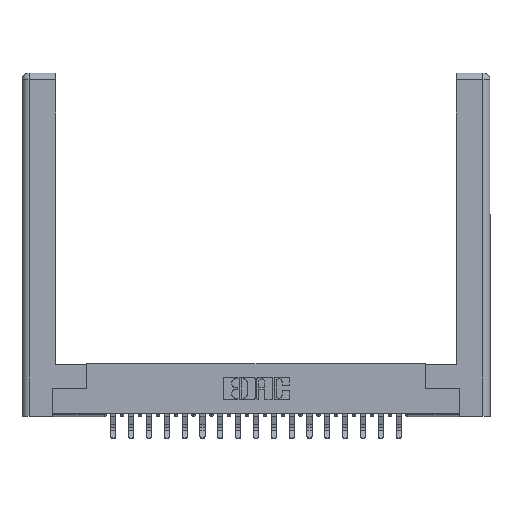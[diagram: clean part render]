
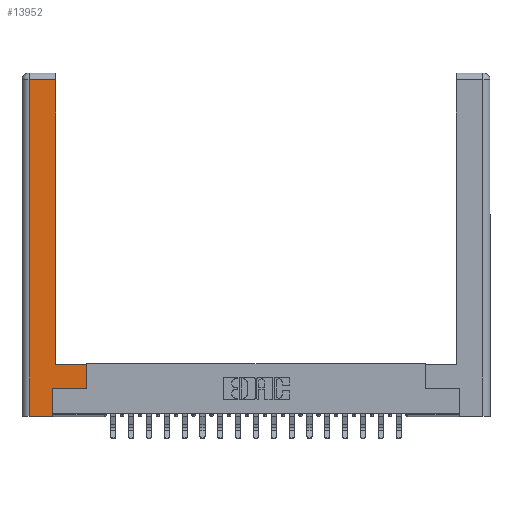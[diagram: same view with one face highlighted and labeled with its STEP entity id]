
A CAD part, top view. The second image highlights one B-rep face of the part: STEP entity #13952.
In plain terms, the highlighted planar face has unit normal (0, 0, 1).
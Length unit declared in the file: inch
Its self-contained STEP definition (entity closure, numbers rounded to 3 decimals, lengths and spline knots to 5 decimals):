
#21 = EDGE_CURVE ( 'NONE', #19868, #20368, #8283, .T. ) ;
#364 = DIRECTION ( 'NONE',  ( -1., 0., 0. ) ) ;
#647 = CARTESIAN_POINT ( 'NONE',  ( 0.0615, 0., 0. ) ) ;
#797 = ORIENTED_EDGE ( 'NONE', *, *, #3730, .T. ) ;
#887 = DIRECTION ( 'NONE',  ( 0., -1., 0. ) ) ;
#927 = ORIENTED_EDGE ( 'NONE', *, *, #7291, .T. ) ;
#1254 = EDGE_CURVE ( 'NONE', #12085, #10074, #23178, .T. ) ;
#1780 = CARTESIAN_POINT ( 'NONE',  ( 0.565, 0.45, 0. ) ) ;
#2742 = ORIENTED_EDGE ( 'NONE', *, *, #9369, .T. ) ;
#2904 = CARTESIAN_POINT ( 'NONE',  ( 0.295, 3., 0. ) ) ;
#3161 = DIRECTION ( 'NONE',  ( 0., 1., 0. ) ) ;
#3313 = CARTESIAN_POINT ( 'NONE',  ( 0.295, 2.94, 0. ) ) ;
#3516 = CARTESIAN_POINT ( 'NONE',  ( 0.0615, 0., 0. ) ) ;
#3673 = LINE ( 'NONE', #7377, #7491 ) ;
#3729 = EDGE_CURVE ( 'NONE', #15984, #19868, #7924, .T. ) ;
#3730 = EDGE_CURVE ( 'NONE', #20303, #15984, #16678, .T. ) ;
#4463 = CARTESIAN_POINT ( 'NONE',  ( 0.265, 0.245, 0. ) ) ;
#4568 = VECTOR ( 'NONE', #23417, 39.37008 ) ;
#6004 = CARTESIAN_POINT ( 'NONE',  ( 0., 0., 0. ) ) ;
#6330 = CARTESIAN_POINT ( 'NONE',  ( 0.265, 0., 0. ) ) ;
#7291 = EDGE_CURVE ( 'NONE', #19706, #12085, #3673, .T. ) ;
#7377 = CARTESIAN_POINT ( 'NONE',  ( 0.265, 0.245, 0. ) ) ;
#7491 = VECTOR ( 'NONE', #22975, 39.37008 ) ;
#7568 = CARTESIAN_POINT ( 'NONE',  ( 0.565, 0.245, 0. ) ) ;
#7638 = DIRECTION ( 'NONE',  ( 1., 0., 0. ) ) ;
#7924 = LINE ( 'NONE', #10699, #23725 ) ;
#8283 = LINE ( 'NONE', #647, #16761 ) ;
#9369 = EDGE_CURVE ( 'NONE', #19134, #20303, #10559, .T. ) ;
#9466 = VECTOR ( 'NONE', #23422, 39.37008 ) ;
#9944 = VECTOR ( 'NONE', #3161, 39.37008 ) ;
#9997 = EDGE_CURVE ( 'NONE', #20368, #19706, #22728, .T. ) ;
#10031 = LINE ( 'NONE', #23668, #9466 ) ;
#10074 = VERTEX_POINT ( 'NONE', #16698 ) ;
#10559 = LINE ( 'NONE', #20299, #12303 ) ;
#10699 = CARTESIAN_POINT ( 'NONE',  ( 0.0615, 2.94, 0. ) ) ;
#10972 = DIRECTION ( 'NONE',  ( -1., 0., 0. ) ) ;
#11454 = DIRECTION ( 'NONE',  ( 0., 0., -1. ) ) ;
#11776 = PLANE ( 'NONE',  #24151 ) ;
#12085 = VERTEX_POINT ( 'NONE', #4463 ) ;
#12303 = VECTOR ( 'NONE', #10972, 39.37008 ) ;
#12710 = CARTESIAN_POINT ( 'NONE',  ( 0.0615, 2.94, 0. ) ) ;
#13183 = VECTOR ( 'NONE', #7638, 39.37008 ) ;
#13471 = ORIENTED_EDGE ( 'NONE', *, *, #1254, .T. ) ;
#13952 = ADVANCED_FACE ( 'NONE', ( #21368 ), #11776, .F. ) ;
#15962 = ORIENTED_EDGE ( 'NONE', *, *, #18430, .T. ) ;
#15984 = VERTEX_POINT ( 'NONE', #3313 ) ;
#16678 = LINE ( 'NONE', #2904, #9944 ) ;
#16698 = CARTESIAN_POINT ( 'NONE',  ( 0.565, 0.245, 0. ) ) ;
#16761 = VECTOR ( 'NONE', #887, 39.37008 ) ;
#17154 = CARTESIAN_POINT ( 'NONE',  ( 0.265, 0., 0. ) ) ;
#18430 = EDGE_CURVE ( 'NONE', #10074, #19134, #10031, .T. ) ;
#19134 = VERTEX_POINT ( 'NONE', #1780 ) ;
#19706 = VERTEX_POINT ( 'NONE', #17154 ) ;
#19868 = VERTEX_POINT ( 'NONE', #12710 ) ;
#20299 = CARTESIAN_POINT ( 'NONE',  ( 0.295, 0.45, 0. ) ) ;
#20303 = VERTEX_POINT ( 'NONE', #21862 ) ;
#20368 = VERTEX_POINT ( 'NONE', #3516 ) ;
#21368 = FACE_OUTER_BOUND ( 'NONE', #24258, .T. ) ;
#21815 = ORIENTED_EDGE ( 'NONE', *, *, #9997, .T. ) ;
#21862 = CARTESIAN_POINT ( 'NONE',  ( 0.295, 0.45, 0. ) ) ;
#22728 = LINE ( 'NONE', #6330, #4568 ) ;
#22975 = DIRECTION ( 'NONE',  ( 0., 1., 0. ) ) ;
#23178 = LINE ( 'NONE', #7568, #13183 ) ;
#23417 = DIRECTION ( 'NONE',  ( 1., 0., 0. ) ) ;
#23422 = DIRECTION ( 'NONE',  ( 0., 1., 0. ) ) ;
#23656 = ORIENTED_EDGE ( 'NONE', *, *, #3729, .T. ) ;
#23663 = ORIENTED_EDGE ( 'NONE', *, *, #21, .T. ) ;
#23668 = CARTESIAN_POINT ( 'NONE',  ( 0.565, 0.45, 0. ) ) ;
#23725 = VECTOR ( 'NONE', #23797, 39.37008 ) ;
#23797 = DIRECTION ( 'NONE',  ( -1., 0., 0. ) ) ;
#24151 = AXIS2_PLACEMENT_3D ( 'NONE', #6004, #11454, #364 ) ;
#24258 = EDGE_LOOP ( 'NONE', ( #797, #23656, #23663, #21815, #927, #13471, #15962, #2742 ) ) ;
